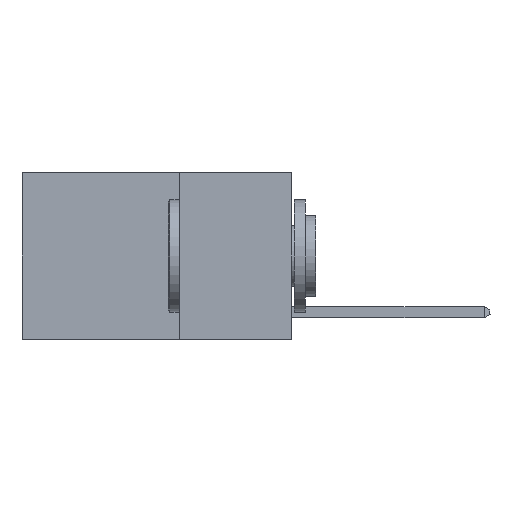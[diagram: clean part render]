
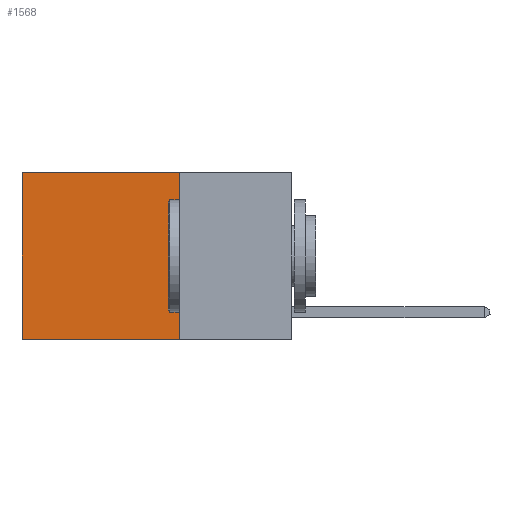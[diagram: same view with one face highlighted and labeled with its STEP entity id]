
A CAD part, left-side view. The second image highlights one B-rep face of the part: STEP entity #1568.
In plain terms, the highlighted planar face has unit normal (-1, 0, 0).
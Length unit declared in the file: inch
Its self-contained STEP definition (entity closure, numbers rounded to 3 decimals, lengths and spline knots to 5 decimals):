
#42 = VERTEX_POINT ( 'NONE', #532 ) ;
#90 = CARTESIAN_POINT ( 'NONE',  ( 0.2625, 0.25, 0. ) ) ;
#532 = CARTESIAN_POINT ( 'NONE',  ( 0.2625, 0.6, 0. ) ) ;
#791 = AXIS2_PLACEMENT_3D ( 'NONE', #90, #12563, #3957 ) ;
#795 = CARTESIAN_POINT ( 'NONE',  ( 0.2625, 0.25, -0.37 ) ) ;
#1018 = ORIENTED_EDGE ( 'NONE', *, *, #11621, .T. ) ;
#1061 = VECTOR ( 'NONE', #6142, 39.37008 ) ;
#1362 = EDGE_CURVE ( 'NONE', #6989, #11380, #11291, .T. ) ;
#1438 = CARTESIAN_POINT ( 'NONE',  ( 0.2625, 0.6, 0. ) ) ;
#1460 = EDGE_LOOP ( 'NONE', ( #10618, #2090, #12116, #1018 ) ) ;
#1568 = ADVANCED_FACE ( 'NONE', ( #12498 ), #4771, .F. ) ;
#2090 = ORIENTED_EDGE ( 'NONE', *, *, #1362, .F. ) ;
#2762 = VERTEX_POINT ( 'NONE', #4840 ) ;
#3957 = DIRECTION ( 'NONE',  ( 0., 0., -1. ) ) ;
#4607 = CARTESIAN_POINT ( 'NONE',  ( 0.2625, 0.25, -0.37 ) ) ;
#4771 = PLANE ( 'NONE',  #791 ) ;
#4840 = CARTESIAN_POINT ( 'NONE',  ( 0.2625, 0.25, 0. ) ) ;
#4954 = EDGE_CURVE ( 'NONE', #2762, #6989, #10027, .T. ) ;
#5975 = LINE ( 'NONE', #10925, #8123 ) ;
#6142 = DIRECTION ( 'NONE',  ( 0., 0., -1. ) ) ;
#6431 = LINE ( 'NONE', #1438, #9908 ) ;
#6989 = VERTEX_POINT ( 'NONE', #4607 ) ;
#7186 = EDGE_CURVE ( 'NONE', #42, #11380, #6431, .T. ) ;
#7397 = CARTESIAN_POINT ( 'NONE',  ( 0.2625, 0.6, -0.37 ) ) ;
#8123 = VECTOR ( 'NONE', #8779, 39.37008 ) ;
#8370 = DIRECTION ( 'NONE',  ( 0., 0., -1. ) ) ;
#8779 = DIRECTION ( 'NONE',  ( 0., 1., 0. ) ) ;
#9494 = DIRECTION ( 'NONE',  ( 0., 1., 0. ) ) ;
#9908 = VECTOR ( 'NONE', #8370, 39.37008 ) ;
#10027 = LINE ( 'NONE', #10797, #1061 ) ;
#10618 = ORIENTED_EDGE ( 'NONE', *, *, #7186, .T. ) ;
#10797 = CARTESIAN_POINT ( 'NONE',  ( 0.2625, 0.25, 0. ) ) ;
#10925 = CARTESIAN_POINT ( 'NONE',  ( 0.2625, 0.25, 0. ) ) ;
#11291 = LINE ( 'NONE', #795, #12460 ) ;
#11380 = VERTEX_POINT ( 'NONE', #7397 ) ;
#11621 = EDGE_CURVE ( 'NONE', #2762, #42, #5975, .T. ) ;
#12116 = ORIENTED_EDGE ( 'NONE', *, *, #4954, .F. ) ;
#12460 = VECTOR ( 'NONE', #9494, 39.37008 ) ;
#12498 = FACE_OUTER_BOUND ( 'NONE', #1460, .T. ) ;
#12563 = DIRECTION ( 'NONE',  ( 1., 0., 0. ) ) ;
